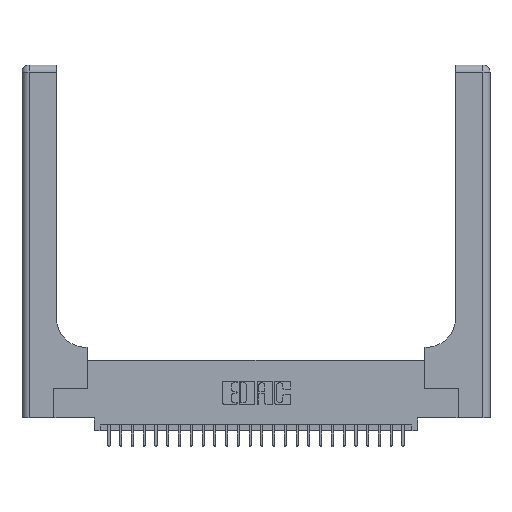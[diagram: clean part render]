
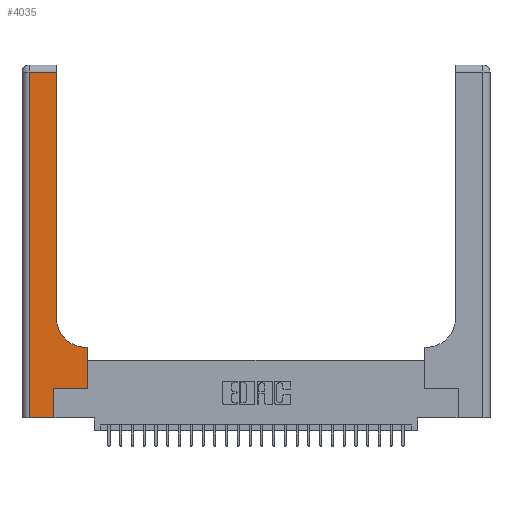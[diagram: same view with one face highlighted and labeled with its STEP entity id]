
A CAD part, top view. The second image highlights one B-rep face of the part: STEP entity #4035.
In plain terms, the highlighted planar face has unit normal (0, 0, 1).
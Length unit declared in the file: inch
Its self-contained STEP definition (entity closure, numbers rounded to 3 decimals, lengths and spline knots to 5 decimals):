
#27 = PLANE ( 'NONE',  #14686 ) ;
#130 = VECTOR ( 'NONE', #25126, 39.37008 ) ;
#505 = EDGE_CURVE ( 'NONE', #11191, #9015, #21310, .T. ) ;
#589 = LINE ( 'NONE', #7097, #11527 ) ;
#642 = AXIS2_PLACEMENT_3D ( 'NONE', #1495, #1088, #9707 ) ;
#1088 = DIRECTION ( 'NONE',  ( 0., 0., -1. ) ) ;
#1276 = VECTOR ( 'NONE', #23754, 39.37008 ) ;
#1495 = CARTESIAN_POINT ( 'NONE',  ( 0.5415, 0.85, 0.37 ) ) ;
#1636 = CARTESIAN_POINT ( 'NONE',  ( 0.269, 0., 0.37 ) ) ;
#2053 = VECTOR ( 'NONE', #5843, 39.37008 ) ;
#2359 = DIRECTION ( 'NONE',  ( 0., 1., 0. ) ) ;
#2544 = VERTEX_POINT ( 'NONE', #7648 ) ;
#2724 = ORIENTED_EDGE ( 'NONE', *, *, #10175, .T. ) ;
#4035 = ADVANCED_FACE ( 'NONE', ( #9208 ), #27, .F. ) ;
#4159 = EDGE_CURVE ( 'NONE', #11291, #11183, #589, .T. ) ;
#4185 = LINE ( 'NONE', #12682, #1276 ) ;
#4224 = CARTESIAN_POINT ( 'NONE',  ( 0.06, 2.94, 0.37 ) ) ;
#4373 = CARTESIAN_POINT ( 'NONE',  ( 0.2915, 3., 0.37 ) ) ;
#5429 = ORIENTED_EDGE ( 'NONE', *, *, #24177, .T. ) ;
#5843 = DIRECTION ( 'NONE',  ( 0., 1., 0. ) ) ;
#5936 = CARTESIAN_POINT ( 'NONE',  ( 0.2915, 2.94, 0.37 ) ) ;
#5967 = LINE ( 'NONE', #14594, #24030 ) ;
#6339 = EDGE_CURVE ( 'NONE', #22697, #13439, #13116, .T. ) ;
#7097 = CARTESIAN_POINT ( 'NONE',  ( 0.06, 3., 0.37 ) ) ;
#7648 = CARTESIAN_POINT ( 'NONE',  ( 0.5585, 0.25, 0.37 ) ) ;
#7832 = VERTEX_POINT ( 'NONE', #15669 ) ;
#8731 = DIRECTION ( 'NONE',  ( 0., 1., 0. ) ) ;
#9015 = VERTEX_POINT ( 'NONE', #22044 ) ;
#9208 = FACE_OUTER_BOUND ( 'NONE', #24534, .T. ) ;
#9707 = DIRECTION ( 'NONE',  ( 1., 0., 0. ) ) ;
#10175 = EDGE_CURVE ( 'NONE', #7832, #15159, #23643, .T. ) ;
#10359 = CARTESIAN_POINT ( 'NONE',  ( 0.5585, 0.25, 0.37 ) ) ;
#11183 = VERTEX_POINT ( 'NONE', #14292 ) ;
#11191 = VERTEX_POINT ( 'NONE', #20682 ) ;
#11291 = VERTEX_POINT ( 'NONE', #4224 ) ;
#11527 = VECTOR ( 'NONE', #18412, 39.37008 ) ;
#12215 = ORIENTED_EDGE ( 'NONE', *, *, #19195, .T. ) ;
#12682 = CARTESIAN_POINT ( 'NONE',  ( 0.269, 0.25, 0.37 ) ) ;
#12779 = ORIENTED_EDGE ( 'NONE', *, *, #6339, .T. ) ;
#12834 = CIRCLE ( 'NONE', #642, 0.25 ) ;
#13116 = LINE ( 'NONE', #23623, #27575 ) ;
#13439 = VERTEX_POINT ( 'NONE', #23727 ) ;
#13469 = DIRECTION ( 'NONE',  ( 0., 0., -1. ) ) ;
#13760 = ORIENTED_EDGE ( 'NONE', *, *, #14809, .T. ) ;
#14292 = CARTESIAN_POINT ( 'NONE',  ( 0.06, 0., 0.37 ) ) ;
#14463 = LINE ( 'NONE', #10359, #2053 ) ;
#14594 = CARTESIAN_POINT ( 'NONE',  ( 0., 2.94, 0.37 ) ) ;
#14686 = AXIS2_PLACEMENT_3D ( 'NONE', #17279, #13469, #15162 ) ;
#14809 = EDGE_CURVE ( 'NONE', #2544, #11191, #14463, .T. ) ;
#15159 = VERTEX_POINT ( 'NONE', #5936 ) ;
#15162 = DIRECTION ( 'NONE',  ( -1., 0., 0. ) ) ;
#15669 = CARTESIAN_POINT ( 'NONE',  ( 0.2915, 0.85, 0.37 ) ) ;
#16067 = ORIENTED_EDGE ( 'NONE', *, *, #4159, .T. ) ;
#16451 = CARTESIAN_POINT ( 'NONE',  ( 0., 0., 0.37 ) ) ;
#17279 = CARTESIAN_POINT ( 'NONE',  ( 0., 3., 0.37 ) ) ;
#18412 = DIRECTION ( 'NONE',  ( 0., -1., 0. ) ) ;
#18915 = CARTESIAN_POINT ( 'NONE',  ( 0.2915, 0.6, 0.37 ) ) ;
#19195 = EDGE_CURVE ( 'NONE', #13439, #2544, #4185, .T. ) ;
#19422 = ORIENTED_EDGE ( 'NONE', *, *, #505, .T. ) ;
#20049 = VECTOR ( 'NONE', #27828, 39.37008 ) ;
#20682 = CARTESIAN_POINT ( 'NONE',  ( 0.5585, 0.6, 0.37 ) ) ;
#20790 = ORIENTED_EDGE ( 'NONE', *, *, #25461, .T. ) ;
#21140 = DIRECTION ( 'NONE',  ( -1., 0., 0. ) ) ;
#21310 = LINE ( 'NONE', #18915, #20049 ) ;
#22044 = CARTESIAN_POINT ( 'NONE',  ( 0.5415, 0.6, 0.37 ) ) ;
#22123 = EDGE_CURVE ( 'NONE', #15159, #11291, #5967, .T. ) ;
#22697 = VERTEX_POINT ( 'NONE', #1636 ) ;
#23163 = VECTOR ( 'NONE', #8731, 39.37008 ) ;
#23623 = CARTESIAN_POINT ( 'NONE',  ( 0.269, 0., 0.37 ) ) ;
#23643 = LINE ( 'NONE', #4373, #23163 ) ;
#23727 = CARTESIAN_POINT ( 'NONE',  ( 0.269, 0.25, 0.37 ) ) ;
#23754 = DIRECTION ( 'NONE',  ( 1., 0., 0. ) ) ;
#24030 = VECTOR ( 'NONE', #21140, 39.37008 ) ;
#24177 = EDGE_CURVE ( 'NONE', #11183, #22697, #27933, .T. ) ;
#24534 = EDGE_LOOP ( 'NONE', ( #2724, #24671, #16067, #5429, #12779, #12215, #13760, #19422, #20790 ) ) ;
#24671 = ORIENTED_EDGE ( 'NONE', *, *, #22123, .T. ) ;
#25126 = DIRECTION ( 'NONE',  ( 1., 0., 0. ) ) ;
#25461 = EDGE_CURVE ( 'NONE', #9015, #7832, #12834, .T. ) ;
#27575 = VECTOR ( 'NONE', #2359, 39.37008 ) ;
#27828 = DIRECTION ( 'NONE',  ( -1., 0., 0. ) ) ;
#27933 = LINE ( 'NONE', #16451, #130 ) ;
